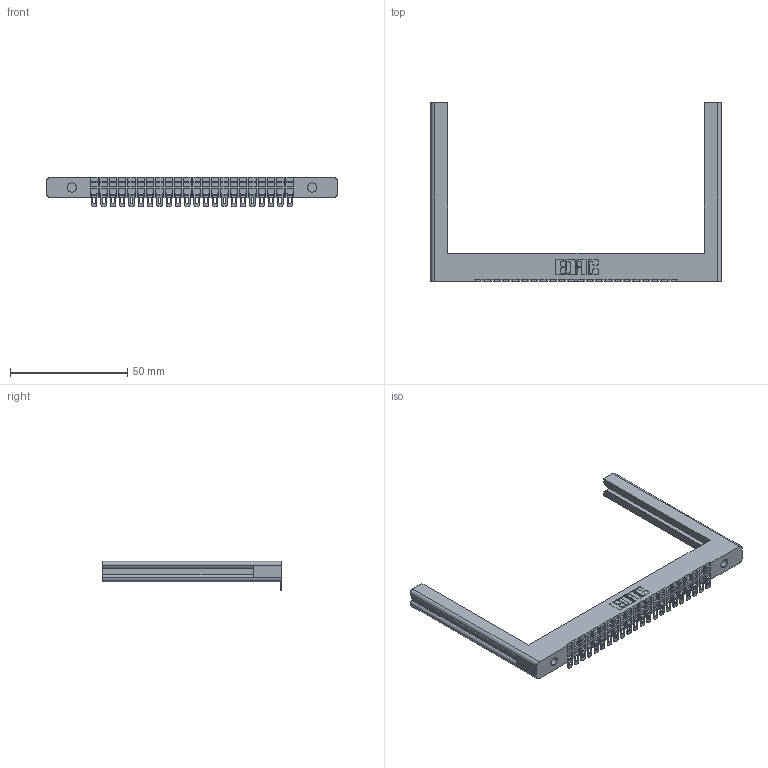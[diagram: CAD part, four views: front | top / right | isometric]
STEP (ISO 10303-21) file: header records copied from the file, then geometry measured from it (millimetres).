
FILE_DESCRIPTION (( 'STEP AP203' ), '1' );
FILE_NAME ('322-022-554-154.STEP', '2018-08-01T11:28:37', ( '' ), ( '' ), 'SwSTEP 2.0', 'SolidWorks 2016', '' );
FILE_SCHEMA (( 'CONFIG_CONTROL_DESIGN' ));
Length unit declared in the file: inch
Products named in the file (3): 322 Part; 307-290-002_554; 322-022-554-154
Assembly tree (23 placements, depth 2):
  322-022-554-154
    322 Part
    307-290-002_554  x22
Bounding box: 123.83 x 76.2 x 12.52 mm (x, y, z)
Volume: 16139 mm3; surface area: 19080.8 mm2
Topology: 23 solids, 23 shells, 1927 faces, 6011 edges, 4006 vertices
Faces by surface type: plane 1235, cylinder 692
Entity records: 23535 total; most frequent: ORIENTED_EDGE 4084, CARTESIAN_POINT 4074, DIRECTION 3636, EDGE_CURVE 2042, LINE 1792, VECTOR 1792, VERTEX_POINT 1360, AXIS2_PLACEMENT_3D 922
